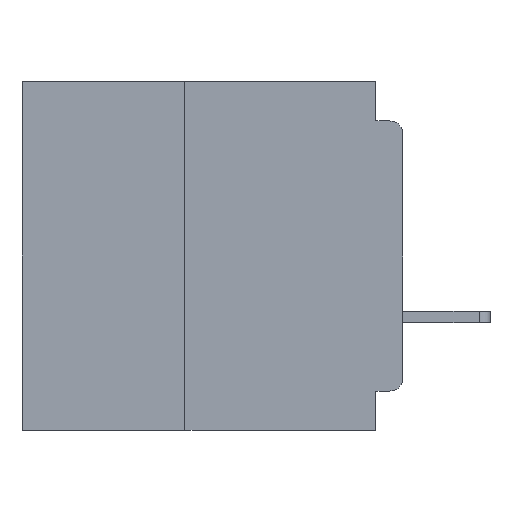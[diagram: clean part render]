
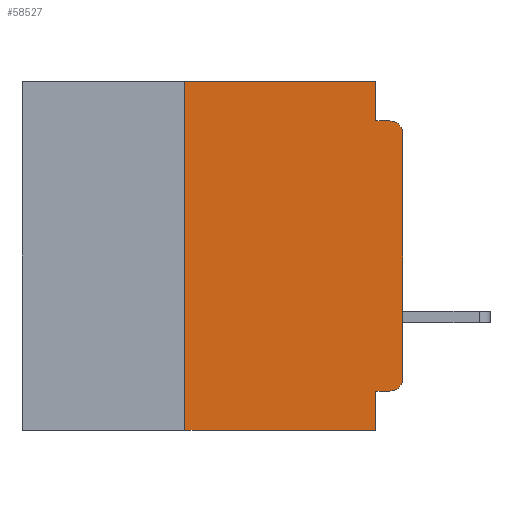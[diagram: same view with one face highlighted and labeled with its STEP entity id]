
A CAD part, left-side view. The second image highlights one B-rep face of the part: STEP entity #58527.
In plain terms, the highlighted planar face has unit normal (-1, 0, 0).
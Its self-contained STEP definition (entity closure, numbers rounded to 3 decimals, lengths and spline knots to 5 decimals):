
#1285 = VERTEX_POINT ( 'NONE', #15300 ) ;
#1538 = AXIS2_PLACEMENT_3D ( 'NONE', #33186, #4356, #37977 ) ;
#1599 = LINE ( 'NONE', #17428, #39959 ) ;
#1986 = ORIENTED_EDGE ( 'NONE', *, *, #6020, .F. ) ;
#2618 = VECTOR ( 'NONE', #16754, 39.37008 ) ;
#2869 = AXIS2_PLACEMENT_3D ( 'NONE', #46579, #17820, #51329 ) ;
#3978 = EDGE_CURVE ( 'NONE', #8661, #35871, #29418, .T. ) ;
#4356 = DIRECTION ( 'NONE',  ( -1., 0., 0. ) ) ;
#5306 = EDGE_CURVE ( 'NONE', #36433, #48065, #1599, .T. ) ;
#5416 = LINE ( 'NONE', #30453, #54870 ) ;
#6020 = EDGE_CURVE ( 'NONE', #26395, #59914, #12119, .T. ) ;
#8376 = CARTESIAN_POINT ( 'NONE',  ( 0., 0., -0.355 ) ) ;
#8661 = VERTEX_POINT ( 'NONE', #12228 ) ;
#9133 = CIRCLE ( 'NONE', #1538, 0.015 ) ;
#10597 = VECTOR ( 'NONE', #41931, 39.37008 ) ;
#12119 = LINE ( 'NONE', #8376, #10597 ) ;
#12228 = CARTESIAN_POINT ( 'NONE',  ( 0., 0., -0.34 ) ) ;
#13904 = LINE ( 'NONE', #59826, #2618 ) ;
#15300 = CARTESIAN_POINT ( 'NONE',  ( 0., 0.031, -0.4 ) ) ;
#15423 = VECTOR ( 'NONE', #61456, 39.37008 ) ;
#15432 = EDGE_CURVE ( 'NONE', #54239, #1285, #45257, .T. ) ;
#16037 = EDGE_CURVE ( 'NONE', #35871, #38275, #39203, .T. ) ;
#16348 = ORIENTED_EDGE ( 'NONE', *, *, #5306, .F. ) ;
#16599 = VECTOR ( 'NONE', #25368, 39.37008 ) ;
#16754 = DIRECTION ( 'NONE',  ( 0., 0., -1. ) ) ;
#17428 = CARTESIAN_POINT ( 'NONE',  ( 0., 0.437, 0. ) ) ;
#17820 = DIRECTION ( 'NONE',  ( 1., 0., 0. ) ) ;
#18316 = CARTESIAN_POINT ( 'NONE',  ( 0., 0.031, -0.045 ) ) ;
#20275 = EDGE_CURVE ( 'NONE', #48065, #60814, #28269, .T. ) ;
#20500 = CARTESIAN_POINT ( 'NONE',  ( 0., 0., 0. ) ) ;
#24514 = EDGE_CURVE ( 'NONE', #59914, #1285, #13904, .T. ) ;
#25368 = DIRECTION ( 'NONE',  ( 0., 0., 1. ) ) ;
#25507 = EDGE_LOOP ( 'NONE', ( #27248, #31447, #58573, #56042, #16348, #52272, #42066, #51303, #1986, #37718 ) ) ;
#26122 = EDGE_CURVE ( 'NONE', #54239, #36433, #5416, .T. ) ;
#26395 = VERTEX_POINT ( 'NONE', #51712 ) ;
#27248 = ORIENTED_EDGE ( 'NONE', *, *, #3978, .T. ) ;
#28096 = DIRECTION ( 'NONE',  ( -1., 0., 0. ) ) ;
#28226 = CARTESIAN_POINT ( 'NONE',  ( 0., 0.25, 0. ) ) ;
#28269 = LINE ( 'NONE', #56684, #15423 ) ;
#28716 = CARTESIAN_POINT ( 'NONE',  ( 0., 0., -0.045 ) ) ;
#28755 = AXIS2_PLACEMENT_3D ( 'NONE', #56661, #28096, #61433 ) ;
#29418 = LINE ( 'NONE', #20500, #16599 ) ;
#30453 = CARTESIAN_POINT ( 'NONE',  ( 0., 0.25, -0.4 ) ) ;
#30670 = DIRECTION ( 'NONE',  ( 0., 0., 1. ) ) ;
#31447 = ORIENTED_EDGE ( 'NONE', *, *, #16037, .T. ) ;
#32171 = PLANE ( 'NONE',  #2869 ) ;
#33186 = CARTESIAN_POINT ( 'NONE',  ( 0., 0.015, -0.34 ) ) ;
#35871 = VERTEX_POINT ( 'NONE', #52502 ) ;
#36369 = VECTOR ( 'NONE', #62062, 39.37008 ) ;
#36433 = VERTEX_POINT ( 'NONE', #28226 ) ;
#37718 = ORIENTED_EDGE ( 'NONE', *, *, #56509, .T. ) ;
#37977 = DIRECTION ( 'NONE',  ( 0., 0., -1. ) ) ;
#38275 = VERTEX_POINT ( 'NONE', #53815 ) ;
#39203 = CIRCLE ( 'NONE', #28755, 0.015 ) ;
#39959 = VECTOR ( 'NONE', #55740, 39.37008 ) ;
#40830 = CARTESIAN_POINT ( 'NONE',  ( 0., 0.031, 0. ) ) ;
#41558 = DIRECTION ( 'NONE',  ( 0., -1., 0. ) ) ;
#41931 = DIRECTION ( 'NONE',  ( 0., 1., 0. ) ) ;
#42066 = ORIENTED_EDGE ( 'NONE', *, *, #15432, .T. ) ;
#45257 = LINE ( 'NONE', #46558, #56422 ) ;
#46558 = CARTESIAN_POINT ( 'NONE',  ( 0., 0.437, -0.4 ) ) ;
#46579 = CARTESIAN_POINT ( 'NONE',  ( 0., 0.437, 0. ) ) ;
#46774 = FACE_OUTER_BOUND ( 'NONE', #25507, .T. ) ;
#48065 = VERTEX_POINT ( 'NONE', #40830 ) ;
#48484 = CARTESIAN_POINT ( 'NONE',  ( 0., 0.25, -0.4 ) ) ;
#49036 = LINE ( 'NONE', #28716, #36369 ) ;
#51303 = ORIENTED_EDGE ( 'NONE', *, *, #24514, .F. ) ;
#51329 = DIRECTION ( 'NONE',  ( 0., 0., -1. ) ) ;
#51639 = EDGE_CURVE ( 'NONE', #60814, #38275, #49036, .T. ) ;
#51712 = CARTESIAN_POINT ( 'NONE',  ( 0., 0.015, -0.355 ) ) ;
#52272 = ORIENTED_EDGE ( 'NONE', *, *, #26122, .F. ) ;
#52502 = CARTESIAN_POINT ( 'NONE',  ( 0., 0., -0.06 ) ) ;
#53815 = CARTESIAN_POINT ( 'NONE',  ( 0., 0.015, -0.045 ) ) ;
#54239 = VERTEX_POINT ( 'NONE', #48484 ) ;
#54870 = VECTOR ( 'NONE', #30670, 39.37008 ) ;
#55740 = DIRECTION ( 'NONE',  ( 0., -1., 0. ) ) ;
#56042 = ORIENTED_EDGE ( 'NONE', *, *, #20275, .F. ) ;
#56422 = VECTOR ( 'NONE', #41558, 39.37008 ) ;
#56509 = EDGE_CURVE ( 'NONE', #26395, #8661, #9133, .T. ) ;
#56661 = CARTESIAN_POINT ( 'NONE',  ( 0., 0.015, -0.06 ) ) ;
#56684 = CARTESIAN_POINT ( 'NONE',  ( 0., 0.031, 0. ) ) ;
#56989 = CARTESIAN_POINT ( 'NONE',  ( 0., 0.031, -0.355 ) ) ;
#58527 = ADVANCED_FACE ( 'NONE', ( #46774 ), #32171, .F. ) ;
#58573 = ORIENTED_EDGE ( 'NONE', *, *, #51639, .F. ) ;
#59826 = CARTESIAN_POINT ( 'NONE',  ( 0., 0.031, -0.4 ) ) ;
#59914 = VERTEX_POINT ( 'NONE', #56989 ) ;
#60814 = VERTEX_POINT ( 'NONE', #18316 ) ;
#61433 = DIRECTION ( 'NONE',  ( 0., 0., -1. ) ) ;
#61456 = DIRECTION ( 'NONE',  ( 0., 0., -1. ) ) ;
#62062 = DIRECTION ( 'NONE',  ( 0., -1., 0. ) ) ;
